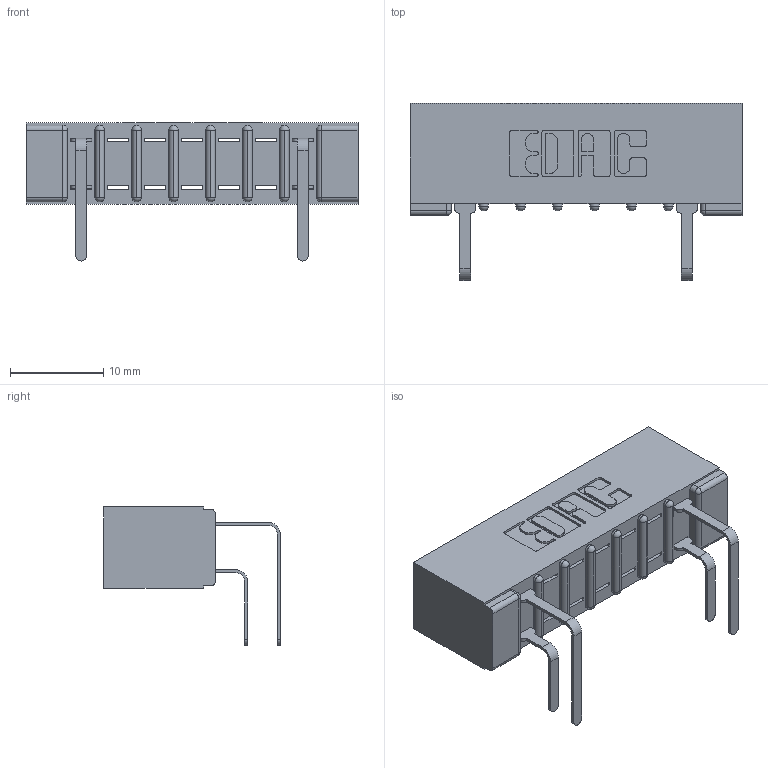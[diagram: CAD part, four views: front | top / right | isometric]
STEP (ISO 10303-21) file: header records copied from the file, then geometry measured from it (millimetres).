
FILE_DESCRIPTION (( 'STEP AP203' ), '1' );
FILE_NAME ('357-007-558-101.STEP', '2018-08-06T23:51:04', ( '' ), ( '' ), 'SwSTEP 2.0', 'SolidWorks 2016', '' );
FILE_SCHEMA (( 'CONFIG_CONTROL_DESIGN' ));
Length unit declared in the file: inch
Products named in the file (4): 357-007-558-101; 307 Part_No Mounting Lugs; 307-290-001_558 559 - 1 (Single); 307-290-001_558 - 2 (Single)
Assembly tree (5 placements, depth 2):
  357-007-558-101
    307 Part_No Mounting Lugs
    307-290-001_558 559 - 1 (Single)  x2
    307-290-001_558 - 2 (Single)  x2
Bounding box: 35.61 x 18.96 x 14.81 mm (x, y, z)
Volume: 2452.4 mm3; surface area: 3355.2 mm2
Topology: 5 solids, 5 shells, 418 faces, 1187 edges, 762 vertices
Faces by surface type: plane 258, cylinder 144, sphere 16
Entity records: 11389 total; most frequent: CARTESIAN_POINT 1915, ORIENTED_EDGE 1902, DIRECTION 1879, EDGE_CURVE 951, VECTOR 715, LINE 715, VERTEX_POINT 618, AXIS2_PLACEMENT_3D 582
